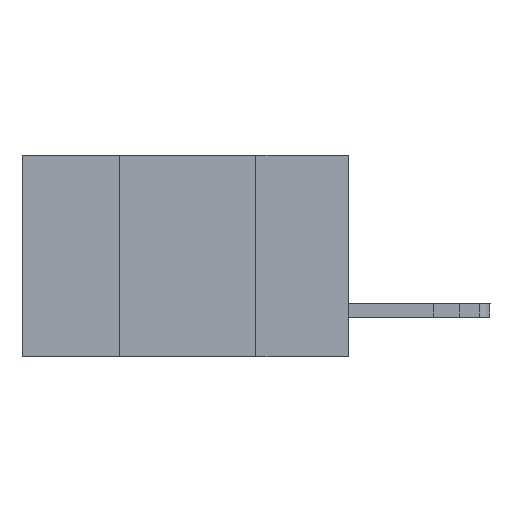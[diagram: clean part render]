
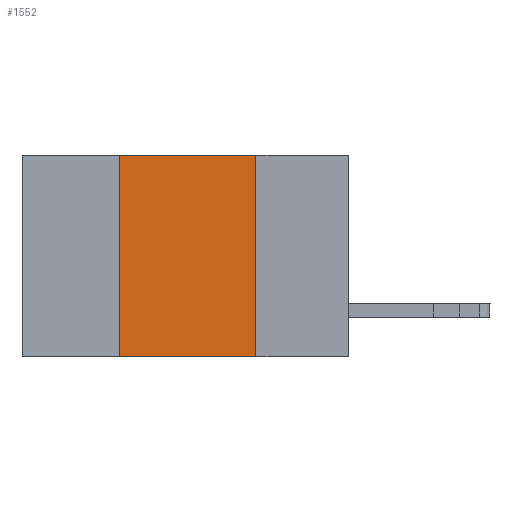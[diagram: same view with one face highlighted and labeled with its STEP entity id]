
A CAD part, left-side view. The second image highlights one B-rep face of the part: STEP entity #1552.
In plain terms, the highlighted planar face has unit normal (-1, 0, 0).
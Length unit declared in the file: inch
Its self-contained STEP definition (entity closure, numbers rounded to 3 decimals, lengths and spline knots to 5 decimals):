
#1053 = DIRECTION ( 'NONE',  ( 0., 0., 1. ) ) ;
#1204 = CARTESIAN_POINT ( 'NONE',  ( 0., 0.42, -0.37 ) ) ;
#1500 = EDGE_CURVE ( 'NONE', #5093, #9264, #2952, .T. ) ;
#1513 = PLANE ( 'NONE',  #7397 ) ;
#1552 = ADVANCED_FACE ( 'NONE', ( #6220 ), #1513, .F. ) ;
#2952 = LINE ( 'NONE', #4716, #9155 ) ;
#3985 = CARTESIAN_POINT ( 'NONE',  ( 0., 0.6, -0.37 ) ) ;
#3998 = VERTEX_POINT ( 'NONE', #1204 ) ;
#4716 = CARTESIAN_POINT ( 'NONE',  ( 0., 0.17, -0.37 ) ) ;
#5030 = DIRECTION ( 'NONE',  ( 1., 0., 0. ) ) ;
#5093 = VERTEX_POINT ( 'NONE', #20312 ) ;
#6220 = FACE_OUTER_BOUND ( 'NONE', #12162, .T. ) ;
#7397 = AXIS2_PLACEMENT_3D ( 'NONE', #19705, #5030, #14556 ) ;
#8209 = DIRECTION ( 'NONE',  ( 0., 0., -1. ) ) ;
#8878 = ORIENTED_EDGE ( 'NONE', *, *, #1500, .F. ) ;
#9155 = VECTOR ( 'NONE', #8209, 39.37008 ) ;
#9264 = VERTEX_POINT ( 'NONE', #10890 ) ;
#10004 = CARTESIAN_POINT ( 'NONE',  ( 0., 0.42, 0. ) ) ;
#10684 = DIRECTION ( 'NONE',  ( 0., -1., 0. ) ) ;
#10890 = CARTESIAN_POINT ( 'NONE',  ( 0., 0.17, -0.37 ) ) ;
#11914 = ORIENTED_EDGE ( 'NONE', *, *, #15166, .F. ) ;
#12162 = EDGE_LOOP ( 'NONE', ( #8878, #11914, #18021, #16118 ) ) ;
#13673 = LINE ( 'NONE', #13889, #19896 ) ;
#13889 = CARTESIAN_POINT ( 'NONE',  ( 0., 0.6, 0. ) ) ;
#13969 = EDGE_CURVE ( 'NONE', #3998, #19698, #20977, .T. ) ;
#14556 = DIRECTION ( 'NONE',  ( 0., 0., -1. ) ) ;
#15166 = EDGE_CURVE ( 'NONE', #19698, #5093, #13673, .T. ) ;
#15606 = LINE ( 'NONE', #3985, #18553 ) ;
#16118 = ORIENTED_EDGE ( 'NONE', *, *, #17303, .T. ) ;
#17303 = EDGE_CURVE ( 'NONE', #3998, #9264, #15606, .T. ) ;
#18021 = ORIENTED_EDGE ( 'NONE', *, *, #13969, .F. ) ;
#18553 = VECTOR ( 'NONE', #10684, 39.37008 ) ;
#19560 = CARTESIAN_POINT ( 'NONE',  ( 0., 0.42, -0.37 ) ) ;
#19698 = VERTEX_POINT ( 'NONE', #10004 ) ;
#19705 = CARTESIAN_POINT ( 'NONE',  ( 0., 0.6, 0. ) ) ;
#19896 = VECTOR ( 'NONE', #20359, 39.37008 ) ;
#20312 = CARTESIAN_POINT ( 'NONE',  ( 0., 0.17, 0. ) ) ;
#20359 = DIRECTION ( 'NONE',  ( 0., -1., 0. ) ) ;
#20548 = VECTOR ( 'NONE', #1053, 39.37008 ) ;
#20977 = LINE ( 'NONE', #19560, #20548 ) ;
